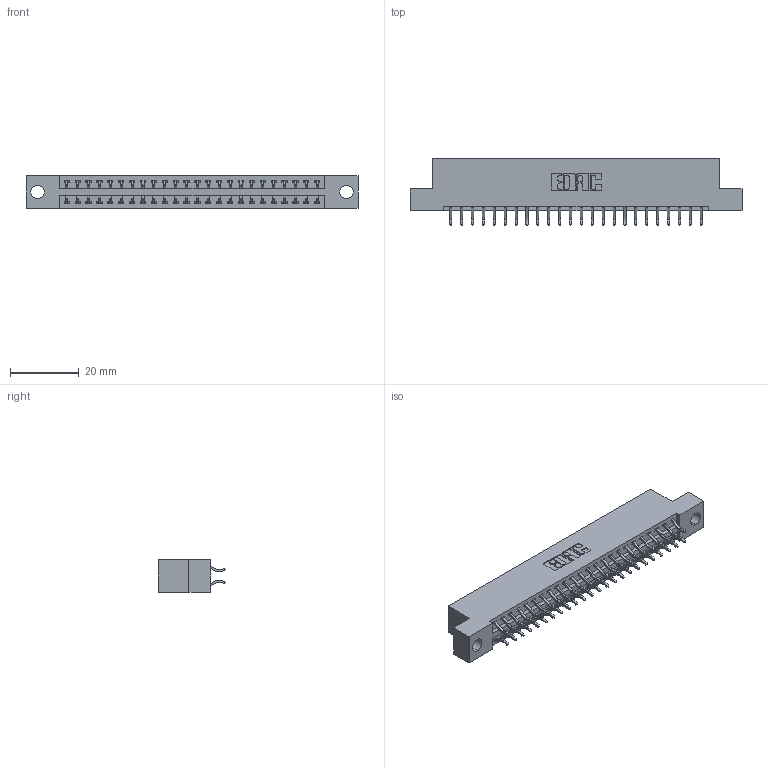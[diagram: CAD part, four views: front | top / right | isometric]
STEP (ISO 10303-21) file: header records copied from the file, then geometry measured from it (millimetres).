
FILE_DESCRIPTION (( 'STEP AP203' ), '1' );
FILE_NAME ('346-048-556-204.STEP', '2022-05-20T21:56:45', ( '' ), ( '' ), 'SwSTEP 2.0', 'SolidWorks 2020', '' );
FILE_SCHEMA (( 'CONFIG_CONTROL_DESIGN' ));
Length unit declared in the file: inch
Products named in the file (3): 346-048-556-204; 345-292-001_556 Tail; 346 Part_Flush Mounting Lugs - 0.156 Dia-TH
Assembly tree (49 placements, depth 2):
  346-048-556-204
    346 Part_Flush Mounting Lugs - 0.156 Dia-TH
    345-292-001_556 Tail  x48
Bounding box: 96.77 x 19.57 x 9.4 mm (x, y, z)
Volume: 9189 mm3; surface area: 12151.3 mm2
Topology: 49 solids, 49 shells, 2920 faces, 8669 edges, 5714 vertices
Faces by surface type: plane 1962, cylinder 958
Entity records: 18725 total; most frequent: CARTESIAN_POINT 3130, ORIENTED_EDGE 3050, DIRECTION 2797, EDGE_CURVE 1525, LINE 1289, VECTOR 1289, VERTEX_POINT 1014, AXIS2_PLACEMENT_3D 754
